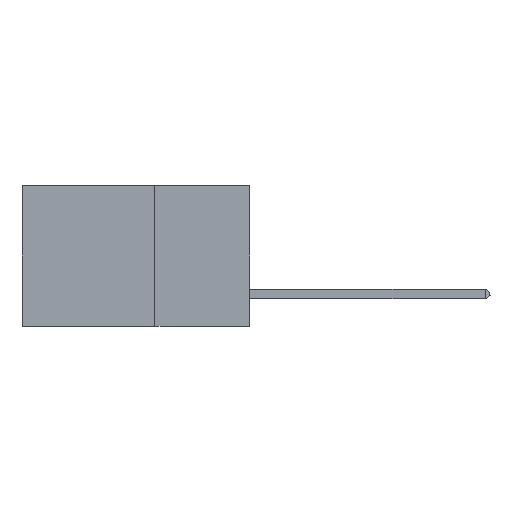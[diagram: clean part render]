
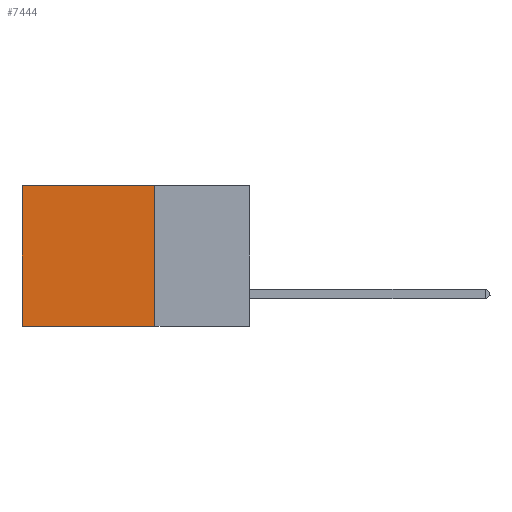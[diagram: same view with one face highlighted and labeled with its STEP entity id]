
A CAD part, left-side view. The second image highlights one B-rep face of the part: STEP entity #7444.
In plain terms, the highlighted planar face has unit normal (-1, 0, 0).
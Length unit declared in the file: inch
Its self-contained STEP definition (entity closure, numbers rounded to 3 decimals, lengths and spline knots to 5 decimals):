
#1449 = PLANE ( 'NONE',  #20722 ) ;
#2329 = DIRECTION ( 'NONE',  ( 0., 1., 0. ) ) ;
#2816 = LINE ( 'NONE', #22991, #23638 ) ;
#4134 = VERTEX_POINT ( 'NONE', #16506 ) ;
#4902 = VERTEX_POINT ( 'NONE', #29913 ) ;
#7444 = ADVANCED_FACE ( 'NONE', ( #41778 ), #1449, .F. ) ;
#7514 = ORIENTED_EDGE ( 'NONE', *, *, #31676, .F. ) ;
#7643 = LINE ( 'NONE', #21151, #22200 ) ;
#9002 = EDGE_CURVE ( 'NONE', #27839, #4134, #2816, .T. ) ;
#10164 = VECTOR ( 'NONE', #31363, 39.37008 ) ;
#10218 = CARTESIAN_POINT ( 'NONE',  ( 0.2875, 0.6, 0. ) ) ;
#11184 = DIRECTION ( 'NONE',  ( 1., 0., 0. ) ) ;
#11413 = CARTESIAN_POINT ( 'NONE',  ( 0.2875, 0.25, 0. ) ) ;
#16273 = EDGE_CURVE ( 'NONE', #4902, #4134, #28323, .T. ) ;
#16506 = CARTESIAN_POINT ( 'NONE',  ( 0.2875, 0.6, -0.37 ) ) ;
#18173 = ORIENTED_EDGE ( 'NONE', *, *, #9002, .T. ) ;
#20455 = DIRECTION ( 'NONE',  ( 0., 0., -1. ) ) ;
#20722 = AXIS2_PLACEMENT_3D ( 'NONE', #11413, #11184, #24702 ) ;
#21151 = CARTESIAN_POINT ( 'NONE',  ( 0.2875, 0.25, 0. ) ) ;
#22200 = VECTOR ( 'NONE', #2329, 39.37008 ) ;
#22991 = CARTESIAN_POINT ( 'NONE',  ( 0.2875, 0.6, 0. ) ) ;
#23638 = VECTOR ( 'NONE', #20455, 39.37008 ) ;
#23703 = VECTOR ( 'NONE', #41631, 39.37008 ) ;
#24184 = CARTESIAN_POINT ( 'NONE',  ( 0.2875, 0.25, 0. ) ) ;
#24695 = LINE ( 'NONE', #24919, #10164 ) ;
#24702 = DIRECTION ( 'NONE',  ( 0., 0., -1. ) ) ;
#24919 = CARTESIAN_POINT ( 'NONE',  ( 0.2875, 0.25, 0. ) ) ;
#27839 = VERTEX_POINT ( 'NONE', #10218 ) ;
#28038 = EDGE_LOOP ( 'NONE', ( #18173, #32898, #7514, #31746 ) ) ;
#28107 = CARTESIAN_POINT ( 'NONE',  ( 0.2875, 0.25, -0.37 ) ) ;
#28323 = LINE ( 'NONE', #28107, #23703 ) ;
#29913 = CARTESIAN_POINT ( 'NONE',  ( 0.2875, 0.25, -0.37 ) ) ;
#31363 = DIRECTION ( 'NONE',  ( 0., 0., -1. ) ) ;
#31676 = EDGE_CURVE ( 'NONE', #40422, #4902, #24695, .T. ) ;
#31746 = ORIENTED_EDGE ( 'NONE', *, *, #31757, .T. ) ;
#31757 = EDGE_CURVE ( 'NONE', #40422, #27839, #7643, .T. ) ;
#32898 = ORIENTED_EDGE ( 'NONE', *, *, #16273, .F. ) ;
#40422 = VERTEX_POINT ( 'NONE', #24184 ) ;
#41631 = DIRECTION ( 'NONE',  ( 0., 1., 0. ) ) ;
#41778 = FACE_OUTER_BOUND ( 'NONE', #28038, .T. ) ;
